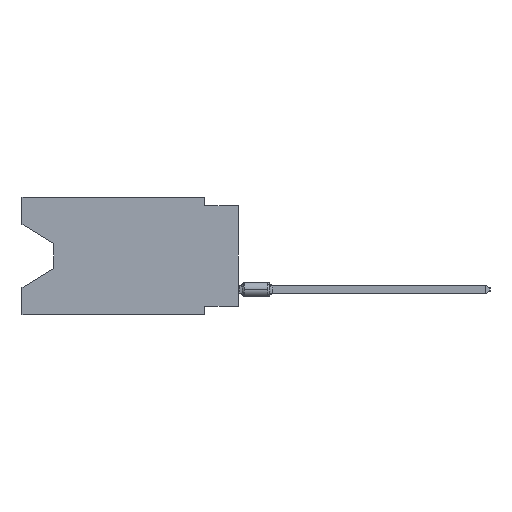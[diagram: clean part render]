
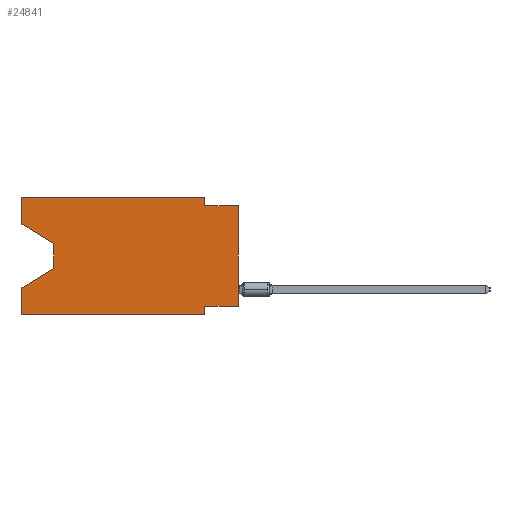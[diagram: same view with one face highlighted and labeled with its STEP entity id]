
A CAD part, left-side view. The second image highlights one B-rep face of the part: STEP entity #24841.
In plain terms, the highlighted planar face has unit normal (-1, 0, 0).
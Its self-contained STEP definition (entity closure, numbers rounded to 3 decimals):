
#366 = EDGE_CURVE ( 'NONE', #21112, #7163, #58552, .T. ) ;
#765 = EDGE_CURVE ( 'NONE', #21112, #26286, #32039, .T. ) ;
#1053 = VERTEX_POINT ( 'NONE', #16946 ) ;
#1130 = LINE ( 'NONE', #28772, #27071 ) ;
#1696 = LINE ( 'NONE', #37383, #56154 ) ;
#2949 = ORIENTED_EDGE ( 'NONE', *, *, #25779, .T. ) ;
#3622 = DIRECTION ( 'NONE',  ( 0., 0., 1. ) ) ;
#4541 = DIRECTION ( 'NONE',  ( 0., -1., 0. ) ) ;
#4919 = AXIS2_PLACEMENT_3D ( 'NONE', #8509, #18010, #26648 ) ;
#4937 = LINE ( 'NONE', #44029, #47140 ) ;
#5450 = VECTOR ( 'NONE', #3622, 1000. ) ;
#6847 = VECTOR ( 'NONE', #23178, 1000. ) ;
#7107 = VERTEX_POINT ( 'NONE', #28948 ) ;
#7163 = VERTEX_POINT ( 'NONE', #51526 ) ;
#8439 = ORIENTED_EDGE ( 'NONE', *, *, #22757, .F. ) ;
#8509 = CARTESIAN_POINT ( 'NONE',  ( 0., 16.383, 0. ) ) ;
#8677 = VECTOR ( 'NONE', #58482, 1000. ) ;
#9373 = CARTESIAN_POINT ( 'NONE',  ( 0., 2.54, -8.89 ) ) ;
#9441 = CARTESIAN_POINT ( 'NONE',  ( 0., 16.383, 0. ) ) ;
#10624 = DIRECTION ( 'NONE',  ( 0., -0.855, -0.519 ) ) ;
#13265 = PLANE ( 'NONE',  #4919 ) ;
#13381 = VECTOR ( 'NONE', #26621, 1000. ) ;
#13727 = LINE ( 'NONE', #26811, #5450 ) ;
#13786 = DIRECTION ( 'NONE',  ( 0., 0., -1. ) ) ;
#13925 = CARTESIAN_POINT ( 'NONE',  ( 0., 2.54, -8.255 ) ) ;
#14981 = ORIENTED_EDGE ( 'NONE', *, *, #35051, .T. ) ;
#15298 = VERTEX_POINT ( 'NONE', #48882 ) ;
#16684 = VERTEX_POINT ( 'NONE', #37340 ) ;
#16946 = CARTESIAN_POINT ( 'NONE',  ( 0., 16.383, -2.038 ) ) ;
#16979 = LINE ( 'NONE', #40451, #49816 ) ;
#18010 = DIRECTION ( 'NONE',  ( 1., 0., 0. ) ) ;
#18029 = CARTESIAN_POINT ( 'NONE',  ( 0., 2.54, -8.89 ) ) ;
#18949 = VECTOR ( 'NONE', #13786, 1000. ) ;
#19607 = VERTEX_POINT ( 'NONE', #18029 ) ;
#21112 = VERTEX_POINT ( 'NONE', #36078 ) ;
#21514 = VERTEX_POINT ( 'NONE', #50566 ) ;
#22205 = ORIENTED_EDGE ( 'NONE', *, *, #38202, .F. ) ;
#22662 = LINE ( 'NONE', #40212, #25620 ) ;
#22757 = EDGE_CURVE ( 'NONE', #15298, #48460, #32210, .T. ) ;
#22947 = VERTEX_POINT ( 'NONE', #39218 ) ;
#23178 = DIRECTION ( 'NONE',  ( 0., 0., 1. ) ) ;
#24841 = ADVANCED_FACE ( 'NONE', ( #35855 ), #13265, .F. ) ;
#25200 = VERTEX_POINT ( 'NONE', #40757 ) ;
#25304 = DIRECTION ( 'NONE',  ( 0., -1., 0. ) ) ;
#25620 = VECTOR ( 'NONE', #4541, 1000. ) ;
#25779 = EDGE_CURVE ( 'NONE', #16684, #22947, #46626, .T. ) ;
#26286 = VERTEX_POINT ( 'NONE', #13925 ) ;
#26621 = DIRECTION ( 'NONE',  ( 0., 0., -1. ) ) ;
#26648 = DIRECTION ( 'NONE',  ( 0., 0., -1. ) ) ;
#26811 = CARTESIAN_POINT ( 'NONE',  ( 0., 16.383, 0. ) ) ;
#27071 = VECTOR ( 'NONE', #37092, 1000. ) ;
#28772 = CARTESIAN_POINT ( 'NONE',  ( 0., 16.383, -8.89 ) ) ;
#28948 = CARTESIAN_POINT ( 'NONE',  ( 0., 16.383, -6.852 ) ) ;
#29989 = EDGE_CURVE ( 'NONE', #22947, #7107, #16979, .T. ) ;
#31224 = CARTESIAN_POINT ( 'NONE',  ( 0., 0., 0. ) ) ;
#31898 = EDGE_CURVE ( 'NONE', #48460, #7163, #4937, .T. ) ;
#31958 = LINE ( 'NONE', #9373, #13381 ) ;
#32039 = LINE ( 'NONE', #35609, #51571 ) ;
#32210 = LINE ( 'NONE', #41423, #18949 ) ;
#33453 = ORIENTED_EDGE ( 'NONE', *, *, #45664, .F. ) ;
#35051 = EDGE_CURVE ( 'NONE', #21514, #19607, #1130, .T. ) ;
#35609 = CARTESIAN_POINT ( 'NONE',  ( 0., 0., -8.255 ) ) ;
#35855 = FACE_OUTER_BOUND ( 'NONE', #56468, .T. ) ;
#36078 = CARTESIAN_POINT ( 'NONE',  ( 0., 0., -8.255 ) ) ;
#37092 = DIRECTION ( 'NONE',  ( 0., -1., 0. ) ) ;
#37340 = CARTESIAN_POINT ( 'NONE',  ( 0., 13.97, -3.505 ) ) ;
#37383 = CARTESIAN_POINT ( 'NONE',  ( 0., 16.383, -2.038 ) ) ;
#38202 = EDGE_CURVE ( 'NONE', #26286, #19607, #31958, .T. ) ;
#38552 = CARTESIAN_POINT ( 'NONE',  ( 0., 13.97, -3.505 ) ) ;
#38876 = ORIENTED_EDGE ( 'NONE', *, *, #31898, .F. ) ;
#39019 = EDGE_CURVE ( 'NONE', #1053, #25200, #54618, .T. ) ;
#39182 = EDGE_CURVE ( 'NONE', #1053, #16684, #1696, .T. ) ;
#39218 = CARTESIAN_POINT ( 'NONE',  ( 0., 13.97, -5.385 ) ) ;
#40212 = CARTESIAN_POINT ( 'NONE',  ( 0., 16.383, 0. ) ) ;
#40451 = CARTESIAN_POINT ( 'NONE',  ( 0., 13.97, -5.385 ) ) ;
#40757 = CARTESIAN_POINT ( 'NONE',  ( 0., 16.383, 0. ) ) ;
#41423 = CARTESIAN_POINT ( 'NONE',  ( 0., 2.54, 0. ) ) ;
#43917 = ORIENTED_EDGE ( 'NONE', *, *, #54778, .F. ) ;
#44029 = CARTESIAN_POINT ( 'NONE',  ( 0., 0., -0.635 ) ) ;
#44470 = CARTESIAN_POINT ( 'NONE',  ( 0., 2.54, -0.635 ) ) ;
#44929 = DIRECTION ( 'NONE',  ( 0., 0.855, -0.519 ) ) ;
#45664 = EDGE_CURVE ( 'NONE', #25200, #15298, #22662, .T. ) ;
#45809 = VECTOR ( 'NONE', #47190, 1000. ) ;
#46626 = LINE ( 'NONE', #38552, #45809 ) ;
#47140 = VECTOR ( 'NONE', #25304, 1000. ) ;
#47190 = DIRECTION ( 'NONE',  ( 0., 0., -1. ) ) ;
#48460 = VERTEX_POINT ( 'NONE', #44470 ) ;
#48882 = CARTESIAN_POINT ( 'NONE',  ( 0., 2.54, 0. ) ) ;
#49014 = ORIENTED_EDGE ( 'NONE', *, *, #765, .F. ) ;
#49816 = VECTOR ( 'NONE', #44929, 1000. ) ;
#50566 = CARTESIAN_POINT ( 'NONE',  ( 0., 16.383, -8.89 ) ) ;
#51526 = CARTESIAN_POINT ( 'NONE',  ( 0., 0., -0.635 ) ) ;
#51571 = VECTOR ( 'NONE', #53729, 1000. ) ;
#53729 = DIRECTION ( 'NONE',  ( 0., 1., 0. ) ) ;
#53754 = ORIENTED_EDGE ( 'NONE', *, *, #366, .T. ) ;
#54618 = LINE ( 'NONE', #9441, #8677 ) ;
#54716 = ORIENTED_EDGE ( 'NONE', *, *, #39182, .T. ) ;
#54778 = EDGE_CURVE ( 'NONE', #21514, #7107, #13727, .T. ) ;
#55100 = ORIENTED_EDGE ( 'NONE', *, *, #39019, .F. ) ;
#55282 = ORIENTED_EDGE ( 'NONE', *, *, #29989, .T. ) ;
#56154 = VECTOR ( 'NONE', #10624, 1000. ) ;
#56468 = EDGE_LOOP ( 'NONE', ( #54716, #2949, #55282, #43917, #14981, #22205, #49014, #53754, #38876, #8439, #33453, #55100 ) ) ;
#58482 = DIRECTION ( 'NONE',  ( 0., 0., 1. ) ) ;
#58552 = LINE ( 'NONE', #31224, #6847 ) ;
